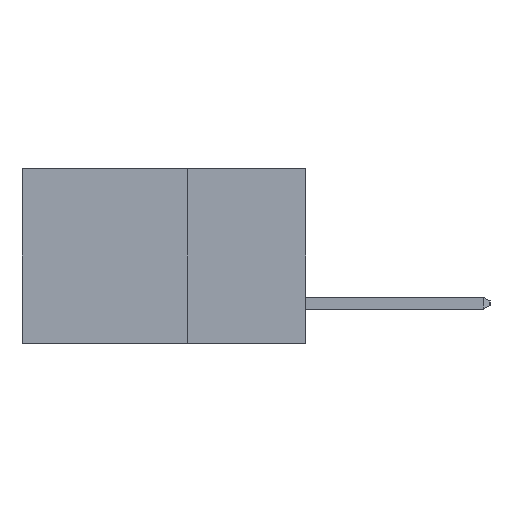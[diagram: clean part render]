
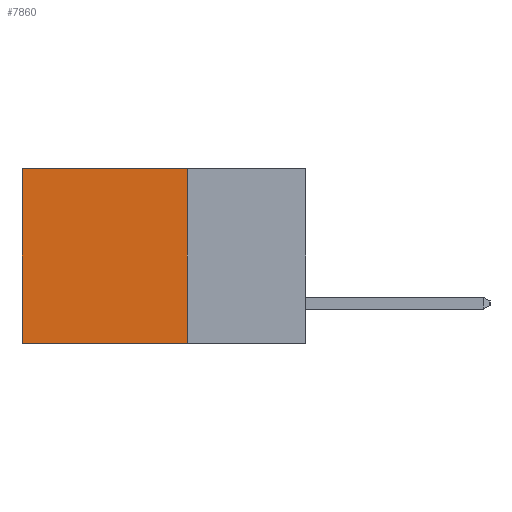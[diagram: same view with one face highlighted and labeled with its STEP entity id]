
A CAD part, left-side view. The second image highlights one B-rep face of the part: STEP entity #7860.
In plain terms, the highlighted planar face has unit normal (-1, 0, 0).
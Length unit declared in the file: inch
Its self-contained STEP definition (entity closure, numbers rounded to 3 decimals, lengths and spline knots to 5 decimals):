
#178 = DIRECTION ( 'NONE',  ( 1., 0., 0. ) ) ;
#549 = DIRECTION ( 'NONE',  ( 0., 0., -1. ) ) ;
#1867 = DIRECTION ( 'NONE',  ( 0., 0., -1. ) ) ;
#2187 = EDGE_LOOP ( 'NONE', ( #9626, #4273, #12180, #8906 ) ) ;
#2213 = FACE_OUTER_BOUND ( 'NONE', #2187, .T. ) ;
#2240 = CARTESIAN_POINT ( 'NONE',  ( 0.298, 0.25, 0. ) ) ;
#2484 = EDGE_CURVE ( 'NONE', #9561, #6921, #2600, .T. ) ;
#2600 = LINE ( 'NONE', #7757, #9846 ) ;
#3147 = LINE ( 'NONE', #9956, #10069 ) ;
#3452 = LINE ( 'NONE', #9356, #8211 ) ;
#3510 = VERTEX_POINT ( 'NONE', #10927 ) ;
#3556 = DIRECTION ( 'NONE',  ( 0., 1., 0. ) ) ;
#3869 = AXIS2_PLACEMENT_3D ( 'NONE', #7804, #178, #6893 ) ;
#4273 = ORIENTED_EDGE ( 'NONE', *, *, #9784, .F. ) ;
#4349 = DIRECTION ( 'NONE',  ( 0., 1., 0. ) ) ;
#4528 = CARTESIAN_POINT ( 'NONE',  ( 0.298, 0.25, -0.37 ) ) ;
#4671 = EDGE_CURVE ( 'NONE', #10419, #3510, #3452, .T. ) ;
#5957 = PLANE ( 'NONE',  #3869 ) ;
#6367 = CARTESIAN_POINT ( 'NONE',  ( 0.298, 0.6, 0. ) ) ;
#6806 = LINE ( 'NONE', #10131, #11453 ) ;
#6893 = DIRECTION ( 'NONE',  ( 0., 0., -1. ) ) ;
#6921 = VERTEX_POINT ( 'NONE', #4528 ) ;
#7368 = EDGE_CURVE ( 'NONE', #9561, #10419, #3147, .T. ) ;
#7757 = CARTESIAN_POINT ( 'NONE',  ( 0.298, 0.25, 0. ) ) ;
#7804 = CARTESIAN_POINT ( 'NONE',  ( 0.298, 0.25, 0. ) ) ;
#7860 = ADVANCED_FACE ( 'NONE', ( #2213 ), #5957, .F. ) ;
#8211 = VECTOR ( 'NONE', #549, 39.37008 ) ;
#8906 = ORIENTED_EDGE ( 'NONE', *, *, #7368, .T. ) ;
#9356 = CARTESIAN_POINT ( 'NONE',  ( 0.298, 0.6, 0. ) ) ;
#9561 = VERTEX_POINT ( 'NONE', #2240 ) ;
#9626 = ORIENTED_EDGE ( 'NONE', *, *, #4671, .T. ) ;
#9784 = EDGE_CURVE ( 'NONE', #6921, #3510, #6806, .T. ) ;
#9846 = VECTOR ( 'NONE', #1867, 39.37008 ) ;
#9956 = CARTESIAN_POINT ( 'NONE',  ( 0.298, 0.25, 0. ) ) ;
#10069 = VECTOR ( 'NONE', #4349, 39.37008 ) ;
#10131 = CARTESIAN_POINT ( 'NONE',  ( 0.298, 0.25, -0.37 ) ) ;
#10419 = VERTEX_POINT ( 'NONE', #6367 ) ;
#10927 = CARTESIAN_POINT ( 'NONE',  ( 0.298, 0.6, -0.37 ) ) ;
#11453 = VECTOR ( 'NONE', #3556, 39.37008 ) ;
#12180 = ORIENTED_EDGE ( 'NONE', *, *, #2484, .F. ) ;
